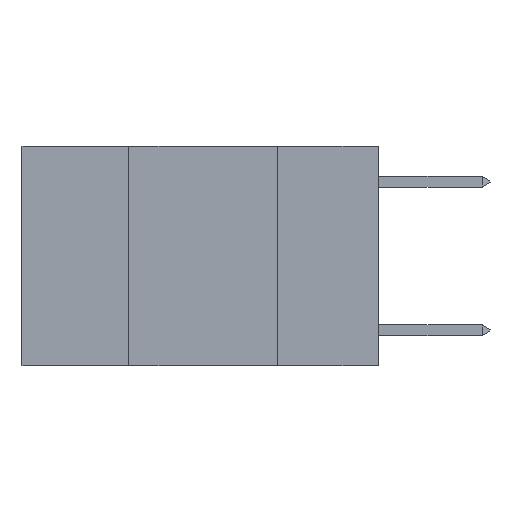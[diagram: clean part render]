
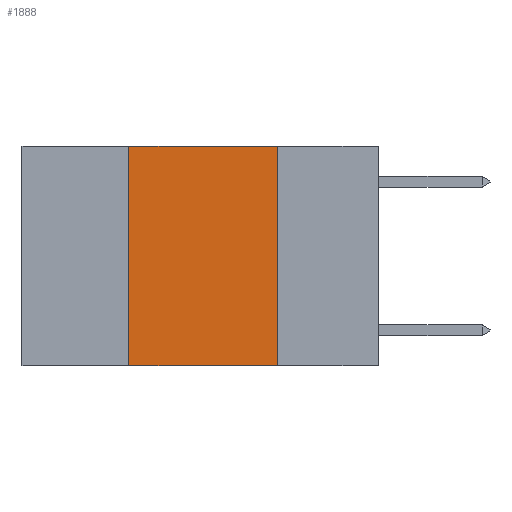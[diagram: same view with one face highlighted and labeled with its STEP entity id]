
A CAD part, left-side view. The second image highlights one B-rep face of the part: STEP entity #1888.
In plain terms, the highlighted planar face has unit normal (-1, 0, 0).
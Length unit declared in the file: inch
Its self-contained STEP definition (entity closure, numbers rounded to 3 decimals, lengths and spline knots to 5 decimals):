
#1492 = EDGE_CURVE ( 'NONE', #2290, #19901, #7116, .T. ) ;
#1888 = ADVANCED_FACE ( 'NONE', ( #14011 ), #2442, .F. ) ;
#2290 = VERTEX_POINT ( 'NONE', #16488 ) ;
#2442 = PLANE ( 'NONE',  #9123 ) ;
#3241 = CARTESIAN_POINT ( 'NONE',  ( 0., 0.42, -0.37 ) ) ;
#3764 = LINE ( 'NONE', #16963, #14782 ) ;
#4058 = CARTESIAN_POINT ( 'NONE',  ( 0., 0.6, 0. ) ) ;
#4242 = EDGE_CURVE ( 'NONE', #8345, #2290, #6635, .T. ) ;
#4959 = CARTESIAN_POINT ( 'NONE',  ( 0., 0.6, -0.37 ) ) ;
#5752 = EDGE_LOOP ( 'NONE', ( #14500, #14951, #6538, #7266 ) ) ;
#6538 = ORIENTED_EDGE ( 'NONE', *, *, #12688, .F. ) ;
#6635 = LINE ( 'NONE', #14845, #14855 ) ;
#7026 = VECTOR ( 'NONE', #13374, 39.37008 ) ;
#7116 = LINE ( 'NONE', #15651, #19139 ) ;
#7266 = ORIENTED_EDGE ( 'NONE', *, *, #20598, .T. ) ;
#8345 = VERTEX_POINT ( 'NONE', #9541 ) ;
#9123 = AXIS2_PLACEMENT_3D ( 'NONE', #4058, #12284, #20511 ) ;
#9541 = CARTESIAN_POINT ( 'NONE',  ( 0., 0.42, 0. ) ) ;
#12284 = DIRECTION ( 'NONE',  ( 1., 0., 0. ) ) ;
#12688 = EDGE_CURVE ( 'NONE', #15653, #8345, #3764, .T. ) ;
#13374 = DIRECTION ( 'NONE',  ( 0., -1., 0. ) ) ;
#13427 = DIRECTION ( 'NONE',  ( 0., -1., 0. ) ) ;
#14011 = FACE_OUTER_BOUND ( 'NONE', #5752, .T. ) ;
#14500 = ORIENTED_EDGE ( 'NONE', *, *, #1492, .F. ) ;
#14782 = VECTOR ( 'NONE', #20530, 39.37008 ) ;
#14845 = CARTESIAN_POINT ( 'NONE',  ( 0., 0.6, 0. ) ) ;
#14855 = VECTOR ( 'NONE', #13427, 39.37008 ) ;
#14951 = ORIENTED_EDGE ( 'NONE', *, *, #4242, .F. ) ;
#15651 = CARTESIAN_POINT ( 'NONE',  ( 0., 0.17, 0. ) ) ;
#15653 = VERTEX_POINT ( 'NONE', #3241 ) ;
#16488 = CARTESIAN_POINT ( 'NONE',  ( 0., 0.17, 0. ) ) ;
#16963 = CARTESIAN_POINT ( 'NONE',  ( 0., 0.42, 0. ) ) ;
#17065 = DIRECTION ( 'NONE',  ( 0., 0., -1. ) ) ;
#19139 = VECTOR ( 'NONE', #17065, 39.37008 ) ;
#19774 = LINE ( 'NONE', #4959, #7026 ) ;
#19901 = VERTEX_POINT ( 'NONE', #20982 ) ;
#20511 = DIRECTION ( 'NONE',  ( 0., 0., -1. ) ) ;
#20530 = DIRECTION ( 'NONE',  ( 0., 0., 1. ) ) ;
#20598 = EDGE_CURVE ( 'NONE', #15653, #19901, #19774, .T. ) ;
#20982 = CARTESIAN_POINT ( 'NONE',  ( 0., 0.17, -0.37 ) ) ;
